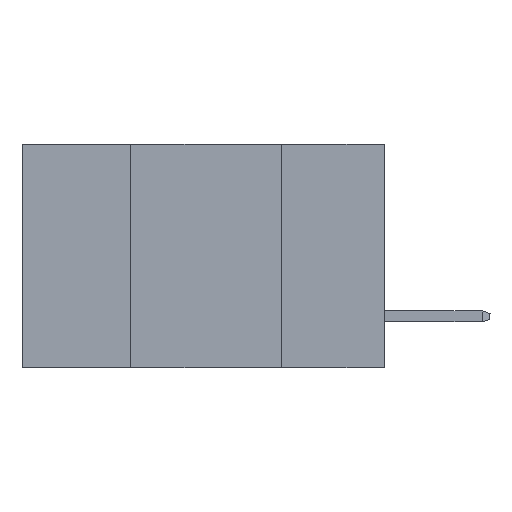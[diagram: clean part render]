
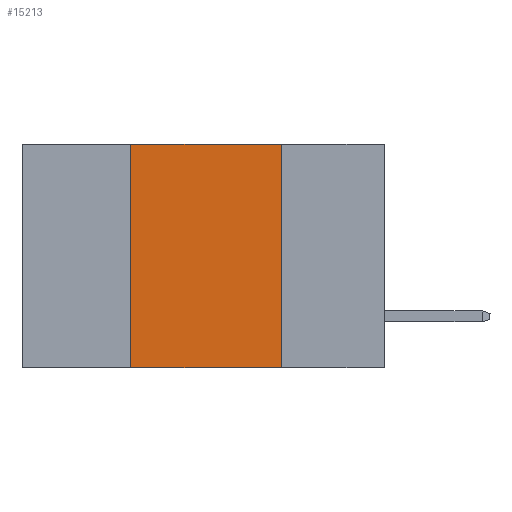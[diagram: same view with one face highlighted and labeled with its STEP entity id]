
A CAD part, left-side view. The second image highlights one B-rep face of the part: STEP entity #15213.
In plain terms, the highlighted planar face has unit normal (-1, 0, 0).
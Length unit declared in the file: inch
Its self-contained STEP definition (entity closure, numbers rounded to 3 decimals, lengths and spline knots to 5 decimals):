
#194 = CARTESIAN_POINT ( 'NONE',  ( 0., 0.42, -0.37 ) ) ;
#298 = VERTEX_POINT ( 'NONE', #7903 ) ;
#1546 = CARTESIAN_POINT ( 'NONE',  ( 0., 0.17, -0.37 ) ) ;
#1948 = EDGE_CURVE ( 'NONE', #298, #12251, #8787, .T. ) ;
#2012 = LINE ( 'NONE', #12377, #14370 ) ;
#2072 = VECTOR ( 'NONE', #6427, 39.37008 ) ;
#2094 = DIRECTION ( 'NONE',  ( 0., 0., 1. ) ) ;
#2427 = EDGE_CURVE ( 'NONE', #10208, #2594, #14436, .T. ) ;
#2594 = VERTEX_POINT ( 'NONE', #1546 ) ;
#3172 = VECTOR ( 'NONE', #10494, 39.37008 ) ;
#3339 = DIRECTION ( 'NONE',  ( 1., 0., 0. ) ) ;
#3456 = ORIENTED_EDGE ( 'NONE', *, *, #1948, .F. ) ;
#4410 = CARTESIAN_POINT ( 'NONE',  ( 0., 0.17, -0.37 ) ) ;
#4670 = CARTESIAN_POINT ( 'NONE',  ( 0., 0.6, 0. ) ) ;
#4840 = CARTESIAN_POINT ( 'NONE',  ( 0., 0.6, -0.37 ) ) ;
#4979 = FACE_OUTER_BOUND ( 'NONE', #10487, .T. ) ;
#6141 = DIRECTION ( 'NONE',  ( 0., 0., -1. ) ) ;
#6427 = DIRECTION ( 'NONE',  ( 0., -1., 0. ) ) ;
#6866 = LINE ( 'NONE', #4410, #7744 ) ;
#7744 = VECTOR ( 'NONE', #10871, 39.37008 ) ;
#7903 = CARTESIAN_POINT ( 'NONE',  ( 0., 0.42, 0. ) ) ;
#8236 = ORIENTED_EDGE ( 'NONE', *, *, #9715, .F. ) ;
#8680 = CARTESIAN_POINT ( 'NONE',  ( 0., 0.6, 0. ) ) ;
#8787 = LINE ( 'NONE', #4670, #3172 ) ;
#9715 = EDGE_CURVE ( 'NONE', #12251, #2594, #6866, .T. ) ;
#10208 = VERTEX_POINT ( 'NONE', #194 ) ;
#10282 = EDGE_CURVE ( 'NONE', #10208, #298, #2012, .T. ) ;
#10487 = EDGE_LOOP ( 'NONE', ( #8236, #3456, #11484, #12979 ) ) ;
#10494 = DIRECTION ( 'NONE',  ( 0., -1., 0. ) ) ;
#10871 = DIRECTION ( 'NONE',  ( 0., 0., -1. ) ) ;
#11484 = ORIENTED_EDGE ( 'NONE', *, *, #10282, .F. ) ;
#12251 = VERTEX_POINT ( 'NONE', #12857 ) ;
#12377 = CARTESIAN_POINT ( 'NONE',  ( 0., 0.42, -0.37 ) ) ;
#12752 = PLANE ( 'NONE',  #16532 ) ;
#12857 = CARTESIAN_POINT ( 'NONE',  ( 0., 0.17, 0. ) ) ;
#12979 = ORIENTED_EDGE ( 'NONE', *, *, #2427, .T. ) ;
#14370 = VECTOR ( 'NONE', #2094, 39.37008 ) ;
#14436 = LINE ( 'NONE', #4840, #2072 ) ;
#15213 = ADVANCED_FACE ( 'NONE', ( #4979 ), #12752, .F. ) ;
#16532 = AXIS2_PLACEMENT_3D ( 'NONE', #8680, #3339, #6141 ) ;
